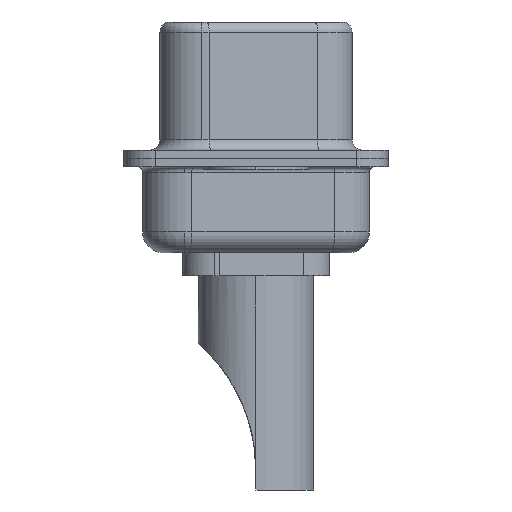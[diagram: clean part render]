
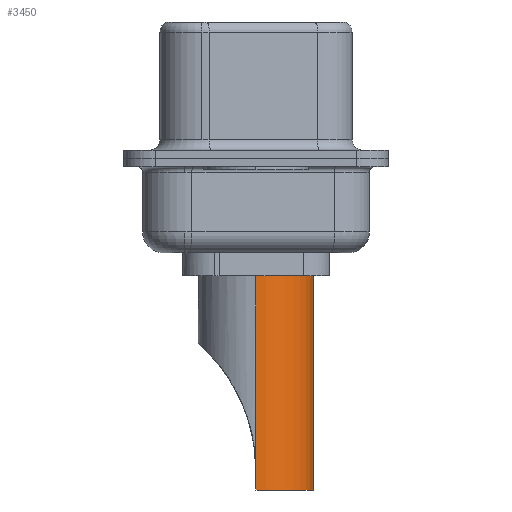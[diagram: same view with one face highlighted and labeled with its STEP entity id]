
A CAD part, left-side view. The second image highlights one B-rep face of the part: STEP entity #3450.
In plain terms, the highlighted cylindrical face has radius 2.75 mm (diameter 5.5 mm), a partial arc.
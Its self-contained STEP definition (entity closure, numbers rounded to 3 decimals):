
#15 = AXIS2_PLACEMENT_3D ( 'NONE', #2300, #9383, #2406 ) ;
#132 = CARTESIAN_POINT ( 'NONE',  ( -2.75, 0., 4.234 ) ) ;
#870 = CARTESIAN_POINT ( 'NONE',  ( -2.75, 0., 1.5 ) ) ;
#1105 = LINE ( 'NONE', #10768, #8113 ) ;
#1358 = EDGE_LOOP ( 'NONE', ( #7863, #5917, #13022, #11375, #3111, #7675 ) ) ;
#1528 = CARTESIAN_POINT ( 'NONE',  ( 0., 0., 1.5 ) ) ;
#2300 = CARTESIAN_POINT ( 'NONE',  ( 0., 0., -8.7 ) ) ;
#2353 = CARTESIAN_POINT ( 'NONE',  ( 2.75, 0., -8.7 ) ) ;
#2406 = DIRECTION ( 'NONE',  ( 1., 0., 0. ) ) ;
#2861 = DIRECTION ( 'NONE',  ( 0., 0., -1. ) ) ;
#3111 = ORIENTED_EDGE ( 'NONE', *, *, #6017, .T. ) ;
#3164 = CYLINDRICAL_SURFACE ( 'NONE', #3897, 2.75 ) ;
#3222 = DIRECTION ( 'NONE',  ( 1., 0., 0. ) ) ;
#3450 = ADVANCED_FACE ( 'NONE', ( #7099 ), #3164, .T. ) ;
#3526 = LINE ( 'NONE', #132, #9751 ) ;
#3719 = CIRCLE ( 'NONE', #4455, 2.75 ) ;
#3897 = AXIS2_PLACEMENT_3D ( 'NONE', #4342, #12437, #3222 ) ;
#4150 = LINE ( 'NONE', #2353, #10763 ) ;
#4180 = DIRECTION ( 'NONE',  ( 0., 0., 1. ) ) ;
#4342 = CARTESIAN_POINT ( 'NONE',  ( 0., 0., 4.234 ) ) ;
#4352 = DIRECTION ( 'NONE',  ( 0., 0., 1. ) ) ;
#4455 = AXIS2_PLACEMENT_3D ( 'NONE', #1528, #10706, #15489 ) ;
#5147 = VERTEX_POINT ( 'NONE', #870 ) ;
#5270 = CARTESIAN_POINT ( 'NONE',  ( -2.75, 0., -8.7 ) ) ;
#5913 = VERTEX_POINT ( 'NONE', #10060 ) ;
#5917 = ORIENTED_EDGE ( 'NONE', *, *, #6099, .T. ) ;
#5987 = EDGE_CURVE ( 'NONE', #5913, #5147, #3526, .T. ) ;
#6017 = EDGE_CURVE ( 'NONE', #10071, #16634, #12853, .T. ) ;
#6099 = EDGE_CURVE ( 'NONE', #5913, #8964, #1105, .T. ) ;
#6102 = EDGE_CURVE ( 'NONE', #8964, #14360, #14588, .T. ) ;
#6126 = EDGE_CURVE ( 'NONE', #10071, #14360, #4150, .T. ) ;
#6148 = EDGE_CURVE ( 'NONE', #5147, #16634, #3719, .T. ) ;
#6501 = CARTESIAN_POINT ( 'NONE',  ( 2.75, 0., -8.7 ) ) ;
#7099 = FACE_OUTER_BOUND ( 'NONE', #1358, .T. ) ;
#7675 = ORIENTED_EDGE ( 'NONE', *, *, #6148, .F. ) ;
#7863 = ORIENTED_EDGE ( 'NONE', *, *, #5987, .F. ) ;
#8113 = VECTOR ( 'NONE', #14645, 1000. ) ;
#8513 = CARTESIAN_POINT ( 'NONE',  ( 2.75, 0., 4.234 ) ) ;
#8964 = VERTEX_POINT ( 'NONE', #5270 ) ;
#9383 = DIRECTION ( 'NONE',  ( 0., 0., 1. ) ) ;
#9751 = VECTOR ( 'NONE', #4352, 1000. ) ;
#9884 = CARTESIAN_POINT ( 'NONE',  ( 2.75, 0., -7.764 ) ) ;
#10060 = CARTESIAN_POINT ( 'NONE',  ( -2.75, 0., -7.764 ) ) ;
#10071 = VERTEX_POINT ( 'NONE', #9884 ) ;
#10706 = DIRECTION ( 'NONE',  ( 0., 0., 1. ) ) ;
#10763 = VECTOR ( 'NONE', #2861, 1000. ) ;
#10768 = CARTESIAN_POINT ( 'NONE',  ( -2.75, 0., -8.7 ) ) ;
#11375 = ORIENTED_EDGE ( 'NONE', *, *, #6126, .F. ) ;
#12437 = DIRECTION ( 'NONE',  ( 0., 0., 1. ) ) ;
#12853 = LINE ( 'NONE', #8513, #13239 ) ;
#13022 = ORIENTED_EDGE ( 'NONE', *, *, #6102, .T. ) ;
#13239 = VECTOR ( 'NONE', #4180, 1000. ) ;
#14360 = VERTEX_POINT ( 'NONE', #6501 ) ;
#14588 = CIRCLE ( 'NONE', #15, 2.75 ) ;
#14645 = DIRECTION ( 'NONE',  ( 0., 0., -1. ) ) ;
#15353 = CARTESIAN_POINT ( 'NONE',  ( 2.75, 0., 1.5 ) ) ;
#15489 = DIRECTION ( 'NONE',  ( 1., 0., 0. ) ) ;
#16634 = VERTEX_POINT ( 'NONE', #15353 ) ;
